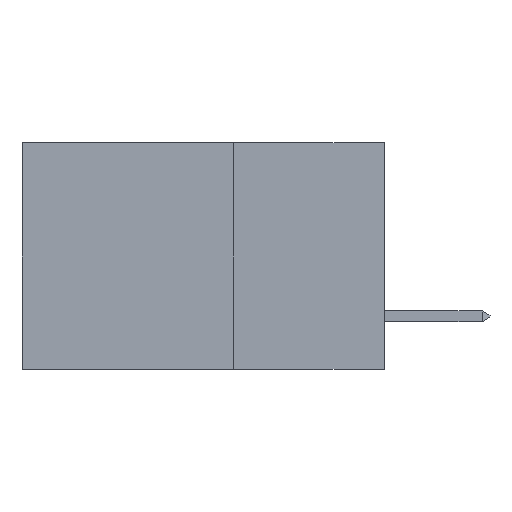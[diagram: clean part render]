
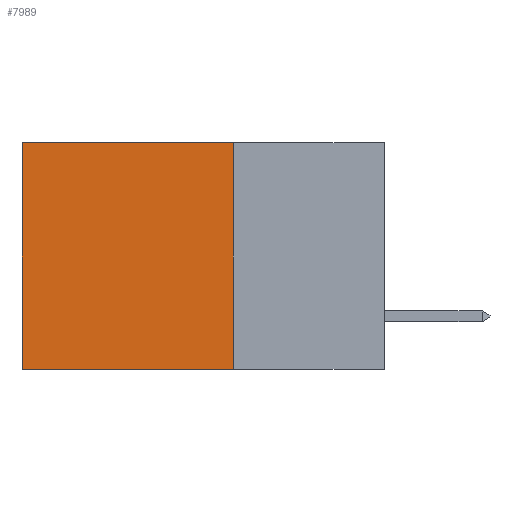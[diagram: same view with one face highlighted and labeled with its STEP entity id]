
A CAD part, left-side view. The second image highlights one B-rep face of the part: STEP entity #7989.
In plain terms, the highlighted planar face has unit normal (-1, 0, 0).
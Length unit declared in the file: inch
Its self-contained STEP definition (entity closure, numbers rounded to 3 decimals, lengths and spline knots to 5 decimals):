
#72 = ORIENTED_EDGE ( 'NONE', *, *, #8083, .F. ) ;
#476 = VERTEX_POINT ( 'NONE', #13011 ) ;
#739 = AXIS2_PLACEMENT_3D ( 'NONE', #6195, #2901, #10722 ) ;
#1792 = LINE ( 'NONE', #9765, #3753 ) ;
#2662 = CARTESIAN_POINT ( 'NONE',  ( 0.2875, 0.25, -0.375 ) ) ;
#2901 = DIRECTION ( 'NONE',  ( 1., 0., 0. ) ) ;
#3043 = DIRECTION ( 'NONE',  ( 0., 0., -1. ) ) ;
#3241 = VECTOR ( 'NONE', #10974, 39.37008 ) ;
#3753 = VECTOR ( 'NONE', #3043, 39.37008 ) ;
#4184 = VECTOR ( 'NONE', #9408, 39.37008 ) ;
#4746 = EDGE_CURVE ( 'NONE', #5890, #7652, #9730, .T. ) ;
#4880 = LINE ( 'NONE', #9340, #13831 ) ;
#5359 = EDGE_CURVE ( 'NONE', #476, #10123, #11749, .T. ) ;
#5890 = VERTEX_POINT ( 'NONE', #2662 ) ;
#6195 = CARTESIAN_POINT ( 'NONE',  ( 0.2875, 0.25, -0.375 ) ) ;
#6366 = ORIENTED_EDGE ( 'NONE', *, *, #4746, .F. ) ;
#6829 = EDGE_CURVE ( 'NONE', #10123, #7652, #1792, .T. ) ;
#7618 = CARTESIAN_POINT ( 'NONE',  ( 0.2875, 0.25, -0.375 ) ) ;
#7652 = VERTEX_POINT ( 'NONE', #9308 ) ;
#7989 = ADVANCED_FACE ( 'NONE', ( #11066 ), #11678, .F. ) ;
#8083 = EDGE_CURVE ( 'NONE', #476, #5890, #4880, .T. ) ;
#8254 = DIRECTION ( 'NONE',  ( 0., 0., -1. ) ) ;
#9308 = CARTESIAN_POINT ( 'NONE',  ( 0.2875, 0.6, -0.375 ) ) ;
#9340 = CARTESIAN_POINT ( 'NONE',  ( 0.2875, 0.25, -0.375 ) ) ;
#9408 = DIRECTION ( 'NONE',  ( 0., 1., 0. ) ) ;
#9730 = LINE ( 'NONE', #7618, #3241 ) ;
#9765 = CARTESIAN_POINT ( 'NONE',  ( 0.2875, 0.6, -0.375 ) ) ;
#10123 = VERTEX_POINT ( 'NONE', #13383 ) ;
#10722 = DIRECTION ( 'NONE',  ( 0., 0., -1. ) ) ;
#10974 = DIRECTION ( 'NONE',  ( 0., 1., 0. ) ) ;
#11066 = FACE_OUTER_BOUND ( 'NONE', #12079, .T. ) ;
#11540 = CARTESIAN_POINT ( 'NONE',  ( 0.2875, 0.25, 0. ) ) ;
#11678 = PLANE ( 'NONE',  #739 ) ;
#11749 = LINE ( 'NONE', #11540, #4184 ) ;
#11799 = ORIENTED_EDGE ( 'NONE', *, *, #6829, .T. ) ;
#12079 = EDGE_LOOP ( 'NONE', ( #11799, #6366, #72, #14354 ) ) ;
#13011 = CARTESIAN_POINT ( 'NONE',  ( 0.2875, 0.25, 0. ) ) ;
#13383 = CARTESIAN_POINT ( 'NONE',  ( 0.2875, 0.6, 0. ) ) ;
#13831 = VECTOR ( 'NONE', #8254, 39.37008 ) ;
#14354 = ORIENTED_EDGE ( 'NONE', *, *, #5359, .T. ) ;
